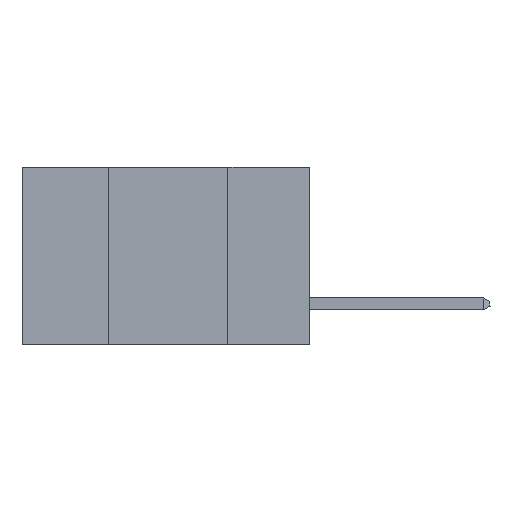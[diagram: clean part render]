
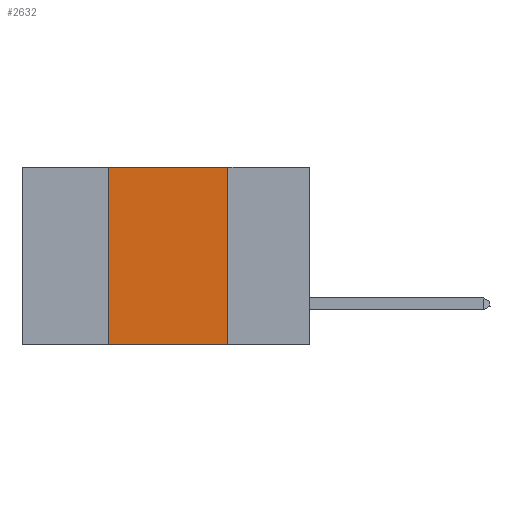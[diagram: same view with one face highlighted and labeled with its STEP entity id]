
A CAD part, left-side view. The second image highlights one B-rep face of the part: STEP entity #2632.
In plain terms, the highlighted planar face has unit normal (-1, 0, 0).
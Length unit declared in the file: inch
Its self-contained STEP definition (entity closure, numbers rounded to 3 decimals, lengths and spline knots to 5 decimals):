
#652 = CARTESIAN_POINT ( 'NONE',  ( 0., 0.17, -0.37 ) ) ;
#971 = DIRECTION ( 'NONE',  ( 0., -1., 0. ) ) ;
#1172 = VERTEX_POINT ( 'NONE', #29904 ) ;
#1482 = LINE ( 'NONE', #11316, #2239 ) ;
#1519 = CARTESIAN_POINT ( 'NONE',  ( 0., 0.42, 0. ) ) ;
#1810 = CARTESIAN_POINT ( 'NONE',  ( 0., 0.6, 0. ) ) ;
#2239 = VECTOR ( 'NONE', #23396, 39.37008 ) ;
#2632 = ADVANCED_FACE ( 'NONE', ( #21484 ), #30377, .F. ) ;
#6332 = CARTESIAN_POINT ( 'NONE',  ( 0., 0.17, 0. ) ) ;
#6978 = LINE ( 'NONE', #13517, #12097 ) ;
#7132 = VERTEX_POINT ( 'NONE', #6332 ) ;
#8583 = DIRECTION ( 'NONE',  ( 0., 0., 1. ) ) ;
#8777 = VERTEX_POINT ( 'NONE', #652 ) ;
#10599 = ORIENTED_EDGE ( 'NONE', *, *, #24520, .T. ) ;
#10905 = LINE ( 'NONE', #26866, #18601 ) ;
#10968 = CARTESIAN_POINT ( 'NONE',  ( 0., 0.42, -0.37 ) ) ;
#11259 = DIRECTION ( 'NONE',  ( 1., 0., 0. ) ) ;
#11316 = CARTESIAN_POINT ( 'NONE',  ( 0., 0.17, 0. ) ) ;
#12097 = VECTOR ( 'NONE', #17978, 39.37008 ) ;
#13517 = CARTESIAN_POINT ( 'NONE',  ( 0., 0.6, -0.37 ) ) ;
#13596 = VERTEX_POINT ( 'NONE', #10968 ) ;
#13894 = EDGE_LOOP ( 'NONE', ( #16825, #25336, #28681, #10599 ) ) ;
#14455 = EDGE_CURVE ( 'NONE', #1172, #7132, #10905, .T. ) ;
#16230 = DIRECTION ( 'NONE',  ( 0., 0., -1. ) ) ;
#16825 = ORIENTED_EDGE ( 'NONE', *, *, #23528, .F. ) ;
#17978 = DIRECTION ( 'NONE',  ( 0., -1., 0. ) ) ;
#18601 = VECTOR ( 'NONE', #971, 39.37008 ) ;
#19833 = LINE ( 'NONE', #1519, #23891 ) ;
#21484 = FACE_OUTER_BOUND ( 'NONE', #13894, .T. ) ;
#23396 = DIRECTION ( 'NONE',  ( 0., 0., -1. ) ) ;
#23528 = EDGE_CURVE ( 'NONE', #7132, #8777, #1482, .T. ) ;
#23891 = VECTOR ( 'NONE', #8583, 39.37008 ) ;
#24520 = EDGE_CURVE ( 'NONE', #13596, #8777, #6978, .T. ) ;
#25336 = ORIENTED_EDGE ( 'NONE', *, *, #14455, .F. ) ;
#26062 = EDGE_CURVE ( 'NONE', #13596, #1172, #19833, .T. ) ;
#26866 = CARTESIAN_POINT ( 'NONE',  ( 0., 0.6, 0. ) ) ;
#27809 = AXIS2_PLACEMENT_3D ( 'NONE', #1810, #11259, #16230 ) ;
#28681 = ORIENTED_EDGE ( 'NONE', *, *, #26062, .F. ) ;
#29904 = CARTESIAN_POINT ( 'NONE',  ( 0., 0.42, 0. ) ) ;
#30377 = PLANE ( 'NONE',  #27809 ) ;
